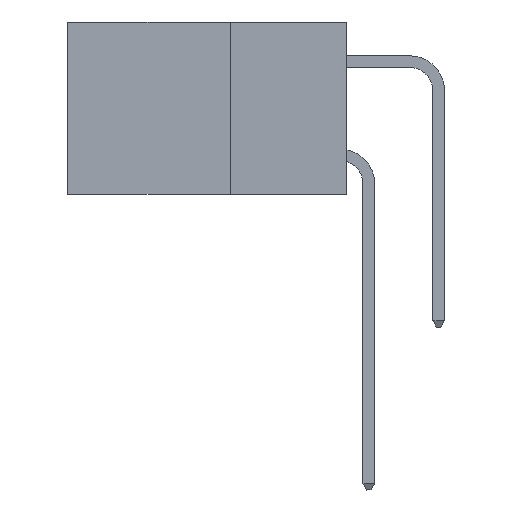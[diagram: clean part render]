
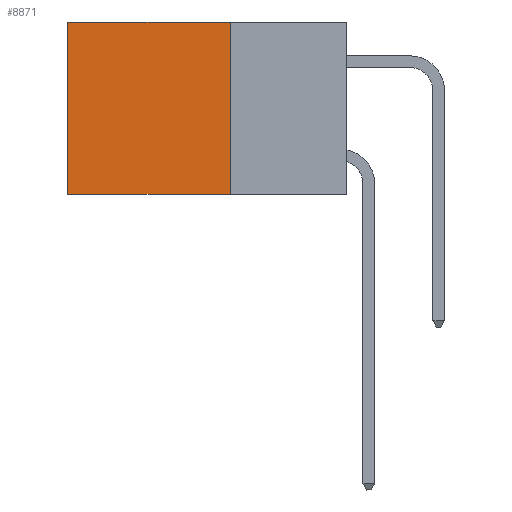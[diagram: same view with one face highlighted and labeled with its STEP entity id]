
A CAD part, left-side view. The second image highlights one B-rep face of the part: STEP entity #8871.
In plain terms, the highlighted planar face has unit normal (-1, 0, 0).
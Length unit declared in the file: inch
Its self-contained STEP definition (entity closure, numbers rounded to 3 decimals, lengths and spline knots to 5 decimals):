
#413 = VERTEX_POINT ( 'NONE', #36674 ) ;
#4335 = LINE ( 'NONE', #17222, #11567 ) ;
#4479 = VERTEX_POINT ( 'NONE', #26533 ) ;
#8474 = CARTESIAN_POINT ( 'NONE',  ( 0.2875, 0.25, -0.37 ) ) ;
#8871 = ADVANCED_FACE ( 'NONE', ( #20784 ), #33567, .F. ) ;
#9105 = ORIENTED_EDGE ( 'NONE', *, *, #12775, .T. ) ;
#11567 = VECTOR ( 'NONE', #23027, 39.37008 ) ;
#11927 = DIRECTION ( 'NONE',  ( 0., 0., -1. ) ) ;
#12775 = EDGE_CURVE ( 'NONE', #22096, #21512, #26298, .T. ) ;
#13217 = ORIENTED_EDGE ( 'NONE', *, *, #30918, .T. ) ;
#13669 = DIRECTION ( 'NONE',  ( 0., 1., 0. ) ) ;
#14544 = CARTESIAN_POINT ( 'NONE',  ( 0.2875, 0.25, 0. ) ) ;
#16498 = DIRECTION ( 'NONE',  ( 0., 0., -1. ) ) ;
#17222 = CARTESIAN_POINT ( 'NONE',  ( 0.2875, 0.6, 0. ) ) ;
#17688 = ORIENTED_EDGE ( 'NONE', *, *, #26461, .F. ) ;
#17930 = VECTOR ( 'NONE', #13669, 39.37008 ) ;
#18175 = DIRECTION ( 'NONE',  ( 1., 0., 0. ) ) ;
#19001 = EDGE_LOOP ( 'NONE', ( #13217, #17688, #23655, #9105 ) ) ;
#20784 = FACE_OUTER_BOUND ( 'NONE', #19001, .T. ) ;
#21512 = VERTEX_POINT ( 'NONE', #32551 ) ;
#22096 = VERTEX_POINT ( 'NONE', #27489 ) ;
#23027 = DIRECTION ( 'NONE',  ( 0., 0., -1. ) ) ;
#23655 = ORIENTED_EDGE ( 'NONE', *, *, #33551, .F. ) ;
#26298 = LINE ( 'NONE', #29290, #17930 ) ;
#26461 = EDGE_CURVE ( 'NONE', #4479, #413, #33106, .T. ) ;
#26533 = CARTESIAN_POINT ( 'NONE',  ( 0.2875, 0.25, -0.37 ) ) ;
#27489 = CARTESIAN_POINT ( 'NONE',  ( 0.2875, 0.25, 0. ) ) ;
#29290 = CARTESIAN_POINT ( 'NONE',  ( 0.2875, 0.25, 0. ) ) ;
#29309 = DIRECTION ( 'NONE',  ( 0., 1., 0. ) ) ;
#30918 = EDGE_CURVE ( 'NONE', #21512, #413, #4335, .T. ) ;
#31448 = VECTOR ( 'NONE', #16498, 39.37008 ) ;
#32244 = AXIS2_PLACEMENT_3D ( 'NONE', #14544, #18175, #11927 ) ;
#32551 = CARTESIAN_POINT ( 'NONE',  ( 0.2875, 0.6, 0. ) ) ;
#33106 = LINE ( 'NONE', #8474, #37909 ) ;
#33551 = EDGE_CURVE ( 'NONE', #22096, #4479, #38088, .T. ) ;
#33567 = PLANE ( 'NONE',  #32244 ) ;
#36674 = CARTESIAN_POINT ( 'NONE',  ( 0.2875, 0.6, -0.37 ) ) ;
#37698 = CARTESIAN_POINT ( 'NONE',  ( 0.2875, 0.25, 0. ) ) ;
#37909 = VECTOR ( 'NONE', #29309, 39.37008 ) ;
#38088 = LINE ( 'NONE', #37698, #31448 ) ;
